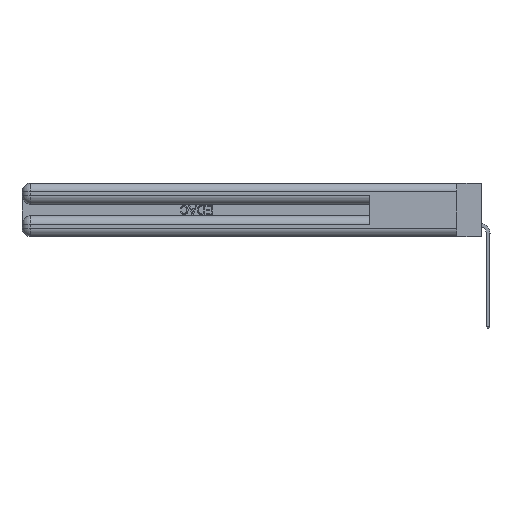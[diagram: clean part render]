
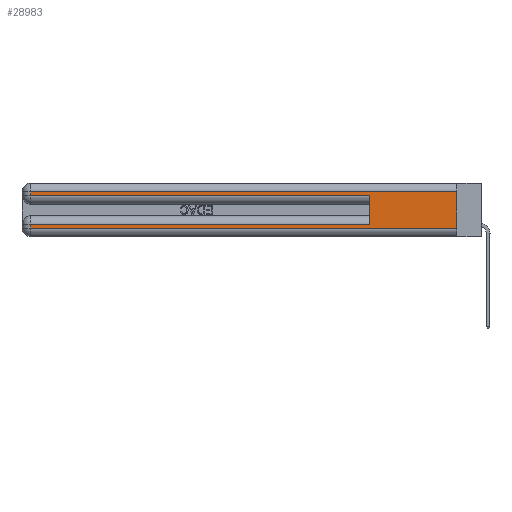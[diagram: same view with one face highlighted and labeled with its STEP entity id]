
A CAD part, left-side view. The second image highlights one B-rep face of the part: STEP entity #28983.
In plain terms, the highlighted planar face has unit normal (-1, 0, 0).
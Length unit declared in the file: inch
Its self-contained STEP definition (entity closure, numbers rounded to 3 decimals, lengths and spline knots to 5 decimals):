
#174 = LINE ( 'NONE', #38387, #21094 ) ;
#936 = LINE ( 'NONE', #36918, #7255 ) ;
#1915 = CARTESIAN_POINT ( 'NONE',  ( 0., 0., 0.31 ) ) ;
#4019 = DIRECTION ( 'NONE',  ( 0., 0., -1. ) ) ;
#5029 = CARTESIAN_POINT ( 'NONE',  ( 0., 2.94, 0.31 ) ) ;
#6999 = CARTESIAN_POINT ( 'NONE',  ( 0., 0., 0.06 ) ) ;
#7005 = VERTEX_POINT ( 'NONE', #1915 ) ;
#7255 = VECTOR ( 'NONE', #16975, 39.37008 ) ;
#8561 = DIRECTION ( 'NONE',  ( 0., 0., -1. ) ) ;
#8734 = PLANE ( 'NONE',  #42957 ) ;
#10113 = VERTEX_POINT ( 'NONE', #6999 ) ;
#10175 = CARTESIAN_POINT ( 'NONE',  ( 0., 2.94, 0.285 ) ) ;
#11467 = EDGE_CURVE ( 'NONE', #33459, #24343, #174, .T. ) ;
#13358 = EDGE_CURVE ( 'NONE', #15502, #31935, #936, .T. ) ;
#13721 = ORIENTED_EDGE ( 'NONE', *, *, #11467, .T. ) ;
#14384 = DIRECTION ( 'NONE',  ( 0., 0., -1. ) ) ;
#14403 = VERTEX_POINT ( 'NONE', #10175 ) ;
#14616 = EDGE_CURVE ( 'NONE', #24343, #10113, #28693, .T. ) ;
#15210 = CARTESIAN_POINT ( 'NONE',  ( 0., 0., 0.06 ) ) ;
#15502 = VERTEX_POINT ( 'NONE', #44418 ) ;
#16055 = DIRECTION ( 'NONE',  ( 0., 1., 0. ) ) ;
#16625 = CARTESIAN_POINT ( 'NONE',  ( 0., 2.94, 0.06 ) ) ;
#16975 = DIRECTION ( 'NONE',  ( 0., 0., 1. ) ) ;
#21094 = VECTOR ( 'NONE', #31689, 39.37008 ) ;
#21126 = ORIENTED_EDGE ( 'NONE', *, *, #35604, .T. ) ;
#21167 = DIRECTION ( 'NONE',  ( 0., -1., 0. ) ) ;
#21352 = VECTOR ( 'NONE', #4019, 39.37008 ) ;
#22051 = EDGE_LOOP ( 'NONE', ( #30244, #21126, #27082, #24082, #45714, #22755, #13721, #24140 ) ) ;
#22412 = LINE ( 'NONE', #37128, #34400 ) ;
#22755 = ORIENTED_EDGE ( 'NONE', *, *, #35689, .T. ) ;
#24082 = ORIENTED_EDGE ( 'NONE', *, *, #35306, .T. ) ;
#24140 = ORIENTED_EDGE ( 'NONE', *, *, #14616, .T. ) ;
#24343 = VERTEX_POINT ( 'NONE', #16625 ) ;
#25371 = LINE ( 'NONE', #37605, #44544 ) ;
#26952 = LINE ( 'NONE', #36765, #21352 ) ;
#27082 = ORIENTED_EDGE ( 'NONE', *, *, #29916, .T. ) ;
#27122 = DIRECTION ( 'NONE',  ( 0., 1., 0. ) ) ;
#28693 = LINE ( 'NONE', #15210, #30296 ) ;
#28983 = ADVANCED_FACE ( 'NONE', ( #36367 ), #8734, .F. ) ;
#29407 = VECTOR ( 'NONE', #14384, 39.37008 ) ;
#29693 = VERTEX_POINT ( 'NONE', #5029 ) ;
#29916 = EDGE_CURVE ( 'NONE', #29693, #14403, #35709, .T. ) ;
#30244 = ORIENTED_EDGE ( 'NONE', *, *, #35981, .F. ) ;
#30296 = VECTOR ( 'NONE', #33415, 39.37008 ) ;
#31036 = VECTOR ( 'NONE', #21167, 39.37008 ) ;
#31689 = DIRECTION ( 'NONE',  ( 0., 0., -1. ) ) ;
#31935 = VERTEX_POINT ( 'NONE', #36602 ) ;
#32520 = CARTESIAN_POINT ( 'NONE',  ( 0., 2.94, 0.085 ) ) ;
#33415 = DIRECTION ( 'NONE',  ( 0., -1., 0. ) ) ;
#33459 = VERTEX_POINT ( 'NONE', #32520 ) ;
#33728 = DIRECTION ( 'NONE',  ( 1., 0., 0. ) ) ;
#34045 = CARTESIAN_POINT ( 'NONE',  ( 0., 0., 0.37 ) ) ;
#34400 = VECTOR ( 'NONE', #27122, 39.37008 ) ;
#35306 = EDGE_CURVE ( 'NONE', #14403, #31935, #40638, .T. ) ;
#35604 = EDGE_CURVE ( 'NONE', #7005, #29693, #22412, .T. ) ;
#35689 = EDGE_CURVE ( 'NONE', #15502, #33459, #25371, .T. ) ;
#35709 = LINE ( 'NONE', #46672, #29407 ) ;
#35981 = EDGE_CURVE ( 'NONE', #7005, #10113, #26952, .T. ) ;
#36367 = FACE_OUTER_BOUND ( 'NONE', #22051, .T. ) ;
#36602 = CARTESIAN_POINT ( 'NONE',  ( 0., 0.6, 0.285 ) ) ;
#36765 = CARTESIAN_POINT ( 'NONE',  ( 0., 0., 0.37 ) ) ;
#36918 = CARTESIAN_POINT ( 'NONE',  ( 0., 0.6, 0.145 ) ) ;
#37128 = CARTESIAN_POINT ( 'NONE',  ( 0., 0., 0.31 ) ) ;
#37605 = CARTESIAN_POINT ( 'NONE',  ( 0., 0., 0.085 ) ) ;
#38387 = CARTESIAN_POINT ( 'NONE',  ( 0., 2.94, 0.37 ) ) ;
#40638 = LINE ( 'NONE', #42872, #31036 ) ;
#42872 = CARTESIAN_POINT ( 'NONE',  ( 0., 0., 0.285 ) ) ;
#42957 = AXIS2_PLACEMENT_3D ( 'NONE', #34045, #33728, #8561 ) ;
#44418 = CARTESIAN_POINT ( 'NONE',  ( 0., 0.6, 0.085 ) ) ;
#44544 = VECTOR ( 'NONE', #16055, 39.37008 ) ;
#45714 = ORIENTED_EDGE ( 'NONE', *, *, #13358, .F. ) ;
#46672 = CARTESIAN_POINT ( 'NONE',  ( 0., 2.94, 0.37 ) ) ;
